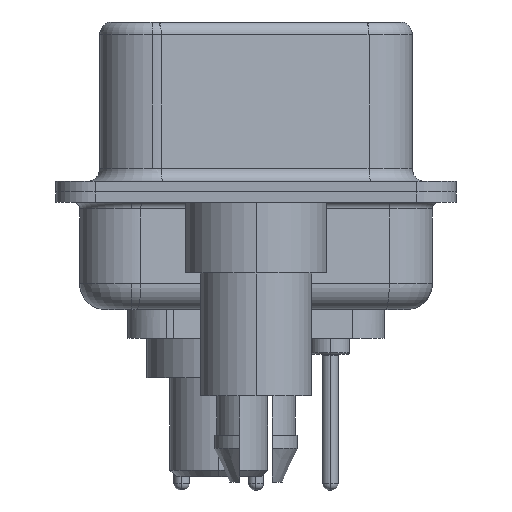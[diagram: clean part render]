
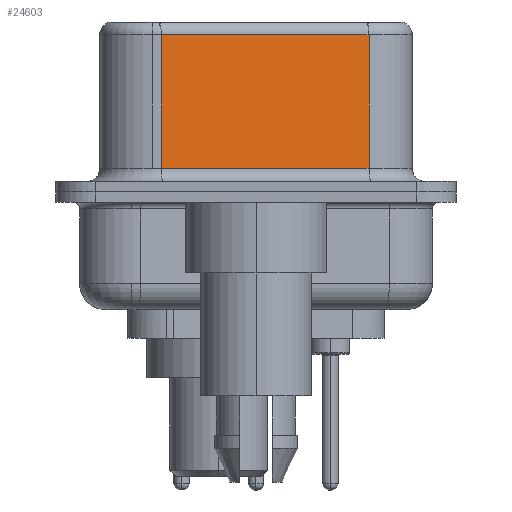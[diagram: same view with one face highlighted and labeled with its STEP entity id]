
A CAD part, left-side view. The second image highlights one B-rep face of the part: STEP entity #24603.
In plain terms, the highlighted planar face has unit normal (-0.985, -0.174, 0).
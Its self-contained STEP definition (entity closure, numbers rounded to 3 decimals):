
#410 = ORIENTED_EDGE ( 'NONE', *, *, #17337, .T. ) ;
#1023 = LINE ( 'NONE', #11113, #6091 ) ;
#1351 = EDGE_CURVE ( 'NONE', #10789, #13712, #17063, .T. ) ;
#2220 = VECTOR ( 'NONE', #23636, 1000. ) ;
#4306 = EDGE_CURVE ( 'NONE', #23803, #13546, #7928, .T. ) ;
#6091 = VECTOR ( 'NONE', #25606, 1000. ) ;
#6886 = DIRECTION ( 'NONE',  ( 0.985, 0.174, 0. ) ) ;
#7928 = LINE ( 'NONE', #14428, #2220 ) ;
#9477 = VECTOR ( 'NONE', #13957, 1000. ) ;
#9634 = DIRECTION ( 'NONE',  ( 0.174, -0.985, 0. ) ) ;
#9759 = LINE ( 'NONE', #20192, #9477 ) ;
#10789 = VERTEX_POINT ( 'NONE', #16568 ) ;
#11113 = CARTESIAN_POINT ( 'NONE',  ( 3.73, 3.628, 6.52 ) ) ;
#12519 = CARTESIAN_POINT ( 'NONE',  ( 5.132, -4.322, 0.9 ) ) ;
#13546 = VERTEX_POINT ( 'NONE', #20898 ) ;
#13712 = VERTEX_POINT ( 'NONE', #23628 ) ;
#13957 = DIRECTION ( 'NONE',  ( 0., 0., -1. ) ) ;
#14428 = CARTESIAN_POINT ( 'NONE',  ( 5.132, -4.322, 6.02 ) ) ;
#15882 = ORIENTED_EDGE ( 'NONE', *, *, #4306, .T. ) ;
#16403 = VECTOR ( 'NONE', #9634, 1000. ) ;
#16568 = CARTESIAN_POINT ( 'NONE',  ( 3.73, 3.628, 0.9 ) ) ;
#17063 = LINE ( 'NONE', #12519, #16403 ) ;
#17337 = EDGE_CURVE ( 'NONE', #13546, #10789, #1023, .T. ) ;
#17702 = AXIS2_PLACEMENT_3D ( 'NONE', #21369, #6886, #21459 ) ;
#19185 = ORIENTED_EDGE ( 'NONE', *, *, #1351, .T. ) ;
#19224 = PLANE ( 'NONE',  #17702 ) ;
#20192 = CARTESIAN_POINT ( 'NONE',  ( 5.132, -4.322, 6.52 ) ) ;
#20898 = CARTESIAN_POINT ( 'NONE',  ( 3.73, 3.628, 6.02 ) ) ;
#21369 = CARTESIAN_POINT ( 'NONE',  ( 5.132, -4.322, 6.52 ) ) ;
#21459 = DIRECTION ( 'NONE',  ( -0.174, 0.985, 0. ) ) ;
#22641 = EDGE_LOOP ( 'NONE', ( #25407, #15882, #410, #19185 ) ) ;
#23628 = CARTESIAN_POINT ( 'NONE',  ( 5.132, -4.322, 0.9 ) ) ;
#23636 = DIRECTION ( 'NONE',  ( -0.174, 0.985, 0. ) ) ;
#23803 = VERTEX_POINT ( 'NONE', #26938 ) ;
#24603 = ADVANCED_FACE ( 'NONE', ( #27069 ), #19224, .F. ) ;
#25407 = ORIENTED_EDGE ( 'NONE', *, *, #25808, .F. ) ;
#25606 = DIRECTION ( 'NONE',  ( 0., 0., -1. ) ) ;
#25808 = EDGE_CURVE ( 'NONE', #23803, #13712, #9759, .T. ) ;
#26938 = CARTESIAN_POINT ( 'NONE',  ( 5.132, -4.322, 6.02 ) ) ;
#27069 = FACE_OUTER_BOUND ( 'NONE', #22641, .T. ) ;
